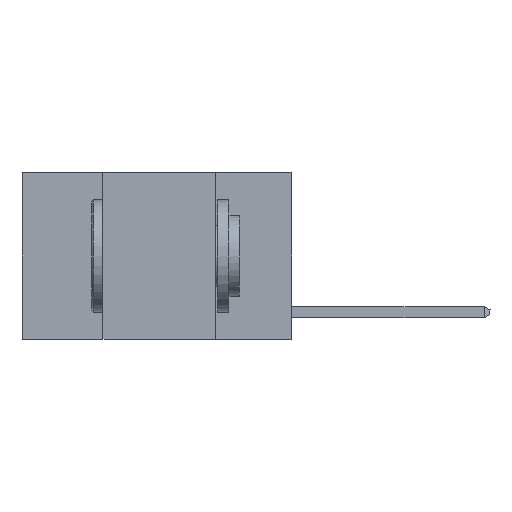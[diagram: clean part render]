
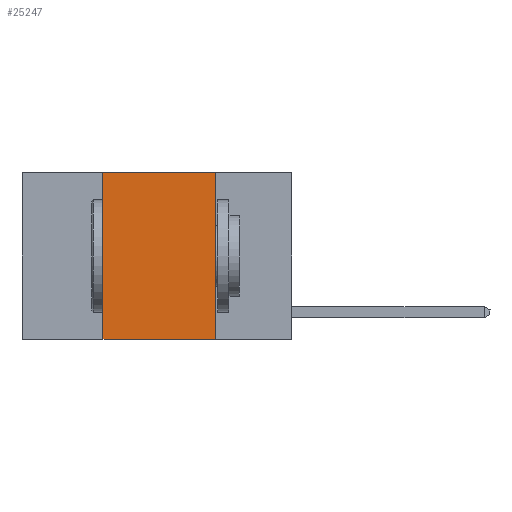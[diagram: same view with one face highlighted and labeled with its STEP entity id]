
A CAD part, left-side view. The second image highlights one B-rep face of the part: STEP entity #25247.
In plain terms, the highlighted planar face has unit normal (-1, 0, 0).
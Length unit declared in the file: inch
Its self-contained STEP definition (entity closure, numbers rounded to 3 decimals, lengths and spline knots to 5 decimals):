
#358 = EDGE_CURVE ( 'NONE', #9069, #3879, #12775, .T. ) ;
#564 = EDGE_CURVE ( 'NONE', #6566, #8876, #26929, .T. ) ;
#927 = DIRECTION ( 'NONE',  ( 0., 0., -1. ) ) ;
#3539 = ORIENTED_EDGE ( 'NONE', *, *, #564, .F. ) ;
#3879 = VERTEX_POINT ( 'NONE', #23853 ) ;
#5587 = DIRECTION ( 'NONE',  ( 1., 0., 0. ) ) ;
#5872 = DIRECTION ( 'NONE',  ( 0., 0., -1. ) ) ;
#6566 = VERTEX_POINT ( 'NONE', #26299 ) ;
#6660 = AXIS2_PLACEMENT_3D ( 'NONE', #26357, #5587, #927 ) ;
#6876 = CARTESIAN_POINT ( 'NONE',  ( 0., 0.42, 0. ) ) ;
#7391 = VECTOR ( 'NONE', #14986, 39.37008 ) ;
#7906 = ORIENTED_EDGE ( 'NONE', *, *, #12048, .F. ) ;
#8876 = VERTEX_POINT ( 'NONE', #6876 ) ;
#9069 = VERTEX_POINT ( 'NONE', #26566 ) ;
#9274 = CARTESIAN_POINT ( 'NONE',  ( 0., 0.6, 0. ) ) ;
#9792 = PLANE ( 'NONE',  #6660 ) ;
#12048 = EDGE_CURVE ( 'NONE', #8876, #9069, #22987, .T. ) ;
#12445 = CARTESIAN_POINT ( 'NONE',  ( 0., 0.6, -0.37 ) ) ;
#12775 = LINE ( 'NONE', #15349, #25989 ) ;
#14986 = DIRECTION ( 'NONE',  ( 0., 0., 1. ) ) ;
#15349 = CARTESIAN_POINT ( 'NONE',  ( 0., 0.17, 0. ) ) ;
#15611 = VECTOR ( 'NONE', #21651, 39.37008 ) ;
#16085 = EDGE_CURVE ( 'NONE', #6566, #3879, #26151, .T. ) ;
#16732 = FACE_OUTER_BOUND ( 'NONE', #18494, .T. ) ;
#18494 = EDGE_LOOP ( 'NONE', ( #24492, #7906, #3539, #20380 ) ) ;
#20380 = ORIENTED_EDGE ( 'NONE', *, *, #16085, .T. ) ;
#21651 = DIRECTION ( 'NONE',  ( 0., -1., 0. ) ) ;
#22551 = DIRECTION ( 'NONE',  ( 0., -1., 0. ) ) ;
#22987 = LINE ( 'NONE', #9274, #23622 ) ;
#23622 = VECTOR ( 'NONE', #22551, 39.37008 ) ;
#23853 = CARTESIAN_POINT ( 'NONE',  ( 0., 0.17, -0.37 ) ) ;
#24492 = ORIENTED_EDGE ( 'NONE', *, *, #358, .F. ) ;
#25247 = ADVANCED_FACE ( 'NONE', ( #16732 ), #9792, .F. ) ;
#25989 = VECTOR ( 'NONE', #5872, 39.37008 ) ;
#26151 = LINE ( 'NONE', #12445, #15611 ) ;
#26299 = CARTESIAN_POINT ( 'NONE',  ( 0., 0.42, -0.37 ) ) ;
#26357 = CARTESIAN_POINT ( 'NONE',  ( 0., 0.6, 0. ) ) ;
#26566 = CARTESIAN_POINT ( 'NONE',  ( 0., 0.17, 0. ) ) ;
#26929 = LINE ( 'NONE', #28517, #7391 ) ;
#28517 = CARTESIAN_POINT ( 'NONE',  ( 0., 0.42, 0. ) ) ;
